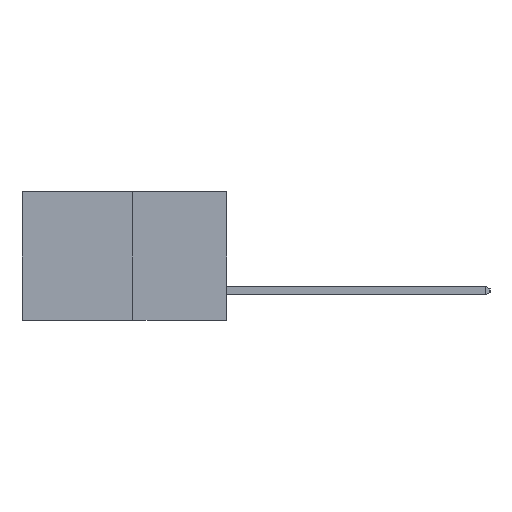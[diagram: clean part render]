
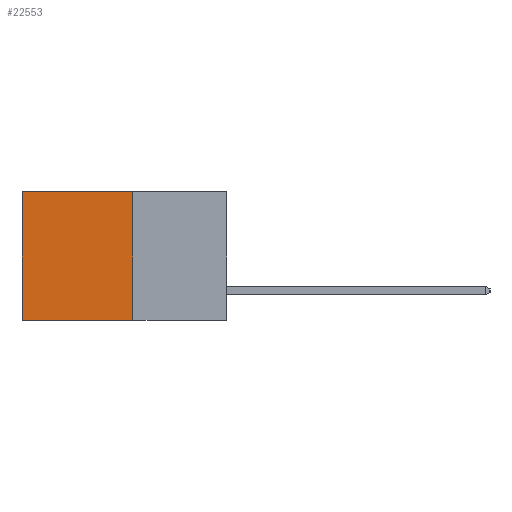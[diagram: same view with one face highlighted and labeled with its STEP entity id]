
A CAD part, left-side view. The second image highlights one B-rep face of the part: STEP entity #22553.
In plain terms, the highlighted planar face has unit normal (-1, 0, 0).
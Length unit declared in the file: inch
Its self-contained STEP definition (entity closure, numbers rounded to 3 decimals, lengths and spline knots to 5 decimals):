
#138 = CARTESIAN_POINT ( 'NONE',  ( 0.277, 0.27, -0.37 ) ) ;
#1725 = CARTESIAN_POINT ( 'NONE',  ( 0.277, 0.27, -0.37 ) ) ;
#1968 = FACE_OUTER_BOUND ( 'NONE', #12699, .T. ) ;
#2473 = VECTOR ( 'NONE', #6993, 39.37008 ) ;
#2722 = CARTESIAN_POINT ( 'NONE',  ( 0.277, 0.59, 0. ) ) ;
#3581 = DIRECTION ( 'NONE',  ( 0., 1., 0. ) ) ;
#4509 = EDGE_CURVE ( 'NONE', #14712, #21222, #8648, .T. ) ;
#6993 = DIRECTION ( 'NONE',  ( 0., 0., -1. ) ) ;
#7095 = EDGE_CURVE ( 'NONE', #16306, #24575, #18615, .T. ) ;
#7432 = CARTESIAN_POINT ( 'NONE',  ( 0.277, 0.27, 0. ) ) ;
#7660 = DIRECTION ( 'NONE',  ( 0., 0., -1. ) ) ;
#8276 = AXIS2_PLACEMENT_3D ( 'NONE', #16257, #24191, #12319 ) ;
#8330 = ORIENTED_EDGE ( 'NONE', *, *, #7095, .T. ) ;
#8362 = PLANE ( 'NONE',  #8276 ) ;
#8569 = VECTOR ( 'NONE', #7660, 39.37008 ) ;
#8648 = LINE ( 'NONE', #16802, #24424 ) ;
#9636 = ORIENTED_EDGE ( 'NONE', *, *, #25553, .F. ) ;
#11614 = CARTESIAN_POINT ( 'NONE',  ( 0.277, 0.27, 0. ) ) ;
#12319 = DIRECTION ( 'NONE',  ( 0., 0., -1. ) ) ;
#12686 = VECTOR ( 'NONE', #3581, 39.37008 ) ;
#12699 = EDGE_LOOP ( 'NONE', ( #13101, #21910, #9636, #8330 ) ) ;
#13101 = ORIENTED_EDGE ( 'NONE', *, *, #18668, .T. ) ;
#14446 = LINE ( 'NONE', #1725, #8569 ) ;
#14712 = VERTEX_POINT ( 'NONE', #138 ) ;
#16257 = CARTESIAN_POINT ( 'NONE',  ( 0.277, 0.27, -0.37 ) ) ;
#16306 = VERTEX_POINT ( 'NONE', #11614 ) ;
#16329 = DIRECTION ( 'NONE',  ( 0., 1., 0. ) ) ;
#16802 = CARTESIAN_POINT ( 'NONE',  ( 0.277, 0.27, -0.37 ) ) ;
#17643 = LINE ( 'NONE', #18857, #2473 ) ;
#18615 = LINE ( 'NONE', #7432, #12686 ) ;
#18668 = EDGE_CURVE ( 'NONE', #24575, #21222, #17643, .T. ) ;
#18857 = CARTESIAN_POINT ( 'NONE',  ( 0.277, 0.59, -0.37 ) ) ;
#21222 = VERTEX_POINT ( 'NONE', #25337 ) ;
#21910 = ORIENTED_EDGE ( 'NONE', *, *, #4509, .F. ) ;
#22553 = ADVANCED_FACE ( 'NONE', ( #1968 ), #8362, .F. ) ;
#24191 = DIRECTION ( 'NONE',  ( 1., 0., 0. ) ) ;
#24424 = VECTOR ( 'NONE', #16329, 39.37008 ) ;
#24575 = VERTEX_POINT ( 'NONE', #2722 ) ;
#25337 = CARTESIAN_POINT ( 'NONE',  ( 0.277, 0.59, -0.37 ) ) ;
#25553 = EDGE_CURVE ( 'NONE', #16306, #14712, #14446, .T. ) ;
